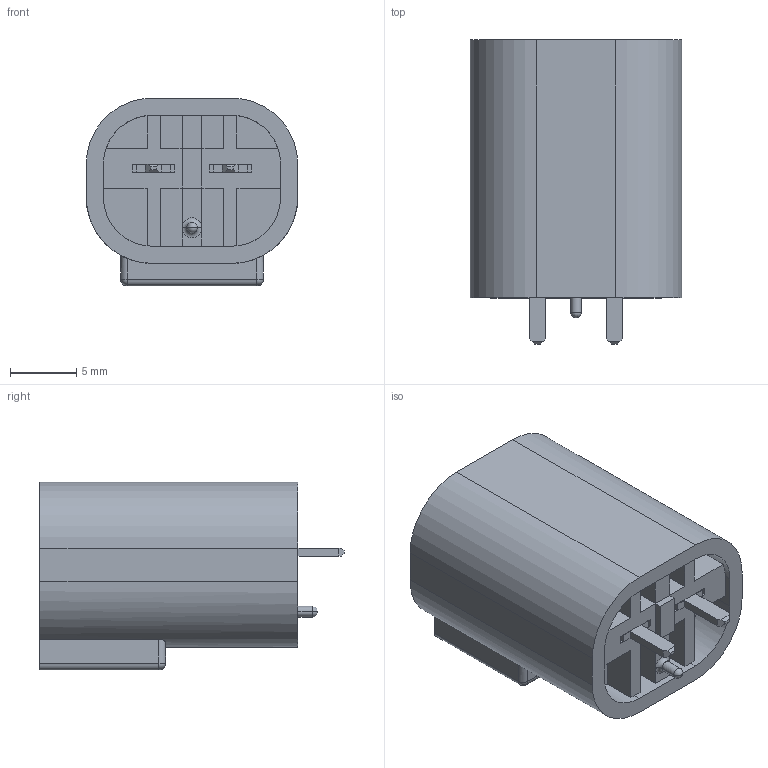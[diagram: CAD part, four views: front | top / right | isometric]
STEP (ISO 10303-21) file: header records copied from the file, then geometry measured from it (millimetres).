
FILE_DESCRIPTION (( 'STEP AP214' ), '1' );
FILE_NAME ('570-002-420-101.STEP', '2020-07-30T14:40:27', ( '' ), ( '' ), 'SwSTEP 2.0', 'SolidWorks 2020', '' );
FILE_SCHEMA (( 'AUTOMOTIVE_DESIGN' ));
Length unit declared in the file: millimetre
Products named in the file (3): 570-002-420-101; 570-002-420-101_Pin; 570-002-420-101_Housing
Assembly tree (3 placements, depth 2):
  570-002-420-101
    570-002-420-101_Housing
    570-002-420-101_Pin  x2
Bounding box: 16 x 23 x 14.2 mm (x, y, z)
Volume: 1547.2 mm3; surface area: 2678.1 mm2
Topology: 3 solids, 3 shells, 213 faces, 577 edges, 369 vertices
Faces by surface type: plane 176, cylinder 25, sphere 4, cone 4, torus 2, bspline 2
Entity records: 5757 total; most frequent: CARTESIAN_POINT 1031, ORIENTED_EDGE 974, DIRECTION 923, EDGE_CURVE 487, LINE 413, VECTOR 413, VERTEX_POINT 311, AXIS2_PLACEMENT_3D 255
